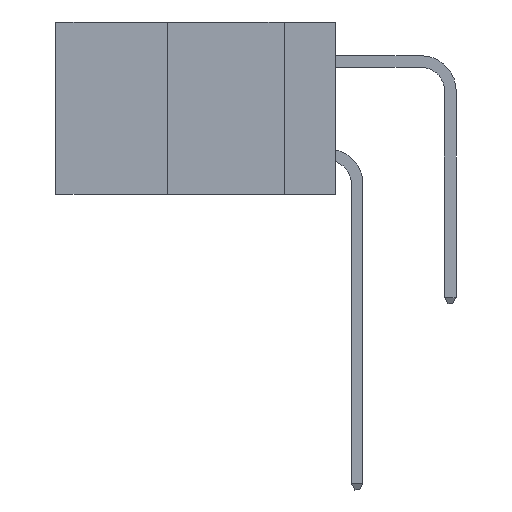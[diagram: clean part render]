
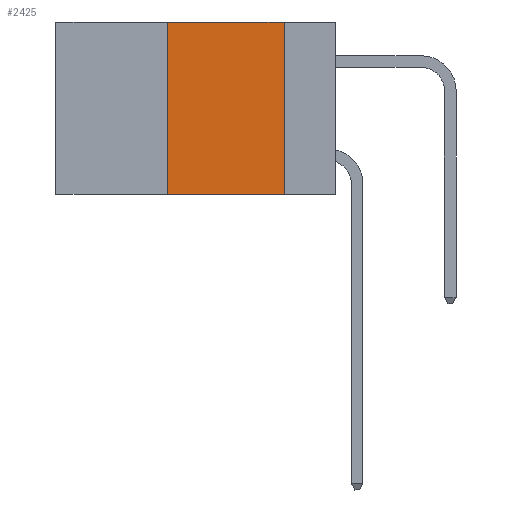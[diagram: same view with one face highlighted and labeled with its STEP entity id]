
A CAD part, left-side view. The second image highlights one B-rep face of the part: STEP entity #2425.
In plain terms, the highlighted planar face has unit normal (-1, 0, 0).
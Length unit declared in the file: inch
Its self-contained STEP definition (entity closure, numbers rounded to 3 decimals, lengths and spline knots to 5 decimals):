
#54 = LINE ( 'NONE', #1568, #15003 ) ;
#522 = EDGE_LOOP ( 'NONE', ( #13013, #5003, #2283, #13910 ) ) ;
#888 = EDGE_CURVE ( 'NONE', #3687, #4171, #54, .T. ) ;
#1568 = CARTESIAN_POINT ( 'NONE',  ( 0., 0.6, 0. ) ) ;
#2283 = ORIENTED_EDGE ( 'NONE', *, *, #11402, .F. ) ;
#2425 = ADVANCED_FACE ( 'NONE', ( #9371 ), #4157, .F. ) ;
#2944 = VECTOR ( 'NONE', #9052, 39.37008 ) ;
#3390 = DIRECTION ( 'NONE',  ( 0., 0., -1. ) ) ;
#3430 = CARTESIAN_POINT ( 'NONE',  ( 0., 0.36, -0.37 ) ) ;
#3687 = VERTEX_POINT ( 'NONE', #14335 ) ;
#4157 = PLANE ( 'NONE',  #14897 ) ;
#4171 = VERTEX_POINT ( 'NONE', #8730 ) ;
#4186 = VERTEX_POINT ( 'NONE', #7495 ) ;
#4302 = EDGE_CURVE ( 'NONE', #12889, #4186, #9830, .T. ) ;
#5003 = ORIENTED_EDGE ( 'NONE', *, *, #888, .F. ) ;
#5846 = DIRECTION ( 'NONE',  ( 0., -1., 0. ) ) ;
#5946 = CARTESIAN_POINT ( 'NONE',  ( 0., 0.6, -0.37 ) ) ;
#6145 = EDGE_CURVE ( 'NONE', #4171, #4186, #14911, .T. ) ;
#6675 = DIRECTION ( 'NONE',  ( 0., -1., 0. ) ) ;
#6710 = VECTOR ( 'NONE', #5846, 39.37008 ) ;
#7081 = CARTESIAN_POINT ( 'NONE',  ( 0., 0.11, 0. ) ) ;
#7495 = CARTESIAN_POINT ( 'NONE',  ( 0., 0.11, -0.37 ) ) ;
#8730 = CARTESIAN_POINT ( 'NONE',  ( 0., 0.11, 0. ) ) ;
#9052 = DIRECTION ( 'NONE',  ( 0., 0., 1. ) ) ;
#9371 = FACE_OUTER_BOUND ( 'NONE', #522, .T. ) ;
#9402 = LINE ( 'NONE', #10196, #2944 ) ;
#9417 = CARTESIAN_POINT ( 'NONE',  ( 0., 0.6, 0. ) ) ;
#9830 = LINE ( 'NONE', #5946, #6710 ) ;
#10196 = CARTESIAN_POINT ( 'NONE',  ( 0., 0.36, 0. ) ) ;
#11402 = EDGE_CURVE ( 'NONE', #12889, #3687, #9402, .T. ) ;
#11943 = VECTOR ( 'NONE', #3390, 39.37008 ) ;
#12889 = VERTEX_POINT ( 'NONE', #3430 ) ;
#13013 = ORIENTED_EDGE ( 'NONE', *, *, #6145, .F. ) ;
#13910 = ORIENTED_EDGE ( 'NONE', *, *, #4302, .T. ) ;
#14189 = DIRECTION ( 'NONE',  ( 0., 0., -1. ) ) ;
#14335 = CARTESIAN_POINT ( 'NONE',  ( 0., 0.36, 0. ) ) ;
#14897 = AXIS2_PLACEMENT_3D ( 'NONE', #9417, #15159, #14189 ) ;
#14911 = LINE ( 'NONE', #7081, #11943 ) ;
#15003 = VECTOR ( 'NONE', #6675, 39.37008 ) ;
#15159 = DIRECTION ( 'NONE',  ( 1., 0., 0. ) ) ;
